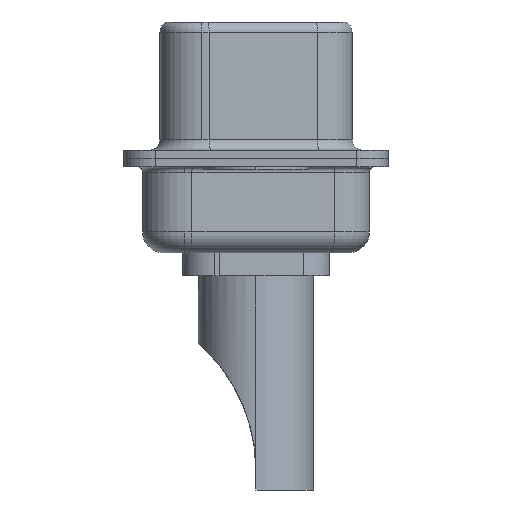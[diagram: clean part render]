
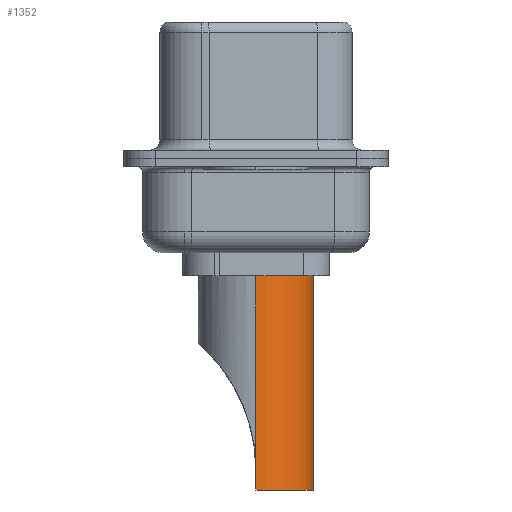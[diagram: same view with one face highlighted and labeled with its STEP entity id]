
A CAD part, left-side view. The second image highlights one B-rep face of the part: STEP entity #1352.
In plain terms, the highlighted cylindrical face has radius 2.75 mm (diameter 5.5 mm), a partial arc.
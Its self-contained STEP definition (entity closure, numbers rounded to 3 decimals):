
#18 = ORIENTED_EDGE ( 'NONE', *, *, #13896, .F. ) ;
#197 = AXIS2_PLACEMENT_3D ( 'NONE', #7029, #8999, #10674 ) ;
#406 = CARTESIAN_POINT ( 'NONE',  ( 2.75, 0., -8.7 ) ) ;
#650 = DIRECTION ( 'NONE',  ( 0., 0., -1. ) ) ;
#826 = DIRECTION ( 'NONE',  ( 1., 0., 0. ) ) ;
#840 = DIRECTION ( 'NONE',  ( 0., 0., 1. ) ) ;
#1222 = ORIENTED_EDGE ( 'NONE', *, *, #8654, .F. ) ;
#1352 = ADVANCED_FACE ( 'NONE', ( #11975 ), #11315, .T. ) ;
#1794 = CARTESIAN_POINT ( 'NONE',  ( 0., 0., 1.5 ) ) ;
#2013 = EDGE_CURVE ( 'NONE', #3887, #9595, #7126, .T. ) ;
#2138 = ORIENTED_EDGE ( 'NONE', *, *, #5776, .T. ) ;
#2928 = DIRECTION ( 'NONE',  ( 1., 0., 0. ) ) ;
#3247 = VERTEX_POINT ( 'NONE', #5244 ) ;
#3299 = DIRECTION ( 'NONE',  ( 0., 0., -1. ) ) ;
#3801 = DIRECTION ( 'NONE',  ( 0., 0., 1. ) ) ;
#3887 = VERTEX_POINT ( 'NONE', #5785 ) ;
#3978 = CARTESIAN_POINT ( 'NONE',  ( -2.75, 0., 4.234 ) ) ;
#4013 = CARTESIAN_POINT ( 'NONE',  ( 2.75, 0., 4.234 ) ) ;
#4053 = ORIENTED_EDGE ( 'NONE', *, *, #2013, .T. ) ;
#4055 = VECTOR ( 'NONE', #650, 1000. ) ;
#4751 = LINE ( 'NONE', #7352, #4055 ) ;
#4976 = EDGE_CURVE ( 'NONE', #8678, #3247, #4751, .T. ) ;
#5244 = CARTESIAN_POINT ( 'NONE',  ( -2.75, 0., -8.7 ) ) ;
#5688 = LINE ( 'NONE', #13472, #13853 ) ;
#5776 = EDGE_CURVE ( 'NONE', #3247, #10967, #6543, .T. ) ;
#5785 = CARTESIAN_POINT ( 'NONE',  ( 2.75, 0., -7.764 ) ) ;
#5970 = VERTEX_POINT ( 'NONE', #7184 ) ;
#6543 = CIRCLE ( 'NONE', #11612, 2.75 ) ;
#6999 = CIRCLE ( 'NONE', #7966, 2.75 ) ;
#7029 = CARTESIAN_POINT ( 'NONE',  ( 0., 0., 4.234 ) ) ;
#7126 = LINE ( 'NONE', #4013, #12445 ) ;
#7179 = ORIENTED_EDGE ( 'NONE', *, *, #7212, .F. ) ;
#7184 = CARTESIAN_POINT ( 'NONE',  ( -2.75, 0., 1.5 ) ) ;
#7212 = EDGE_CURVE ( 'NONE', #3887, #10967, #5688, .T. ) ;
#7331 = DIRECTION ( 'NONE',  ( 0., 0., 1. ) ) ;
#7352 = CARTESIAN_POINT ( 'NONE',  ( -2.75, 0., -8.7 ) ) ;
#7966 = AXIS2_PLACEMENT_3D ( 'NONE', #1794, #9465, #2928 ) ;
#8654 = EDGE_CURVE ( 'NONE', #5970, #9595, #6999, .T. ) ;
#8678 = VERTEX_POINT ( 'NONE', #13681 ) ;
#8762 = CARTESIAN_POINT ( 'NONE',  ( 2.75, 0., 1.5 ) ) ;
#8999 = DIRECTION ( 'NONE',  ( 0., 0., 1. ) ) ;
#9465 = DIRECTION ( 'NONE',  ( 0., 0., 1. ) ) ;
#9595 = VERTEX_POINT ( 'NONE', #8762 ) ;
#10269 = ORIENTED_EDGE ( 'NONE', *, *, #4976, .T. ) ;
#10484 = EDGE_LOOP ( 'NONE', ( #18, #10269, #2138, #7179, #4053, #1222 ) ) ;
#10600 = LINE ( 'NONE', #3978, #13088 ) ;
#10674 = DIRECTION ( 'NONE',  ( 1., 0., 0. ) ) ;
#10967 = VERTEX_POINT ( 'NONE', #406 ) ;
#11315 = CYLINDRICAL_SURFACE ( 'NONE', #197, 2.75 ) ;
#11612 = AXIS2_PLACEMENT_3D ( 'NONE', #12331, #840, #826 ) ;
#11975 = FACE_OUTER_BOUND ( 'NONE', #10484, .T. ) ;
#12331 = CARTESIAN_POINT ( 'NONE',  ( 0., 0., -8.7 ) ) ;
#12445 = VECTOR ( 'NONE', #3801, 1000. ) ;
#13088 = VECTOR ( 'NONE', #7331, 1000. ) ;
#13472 = CARTESIAN_POINT ( 'NONE',  ( 2.75, 0., -8.7 ) ) ;
#13681 = CARTESIAN_POINT ( 'NONE',  ( -2.75, 0., -7.764 ) ) ;
#13853 = VECTOR ( 'NONE', #3299, 1000. ) ;
#13896 = EDGE_CURVE ( 'NONE', #8678, #5970, #10600, .T. ) ;
